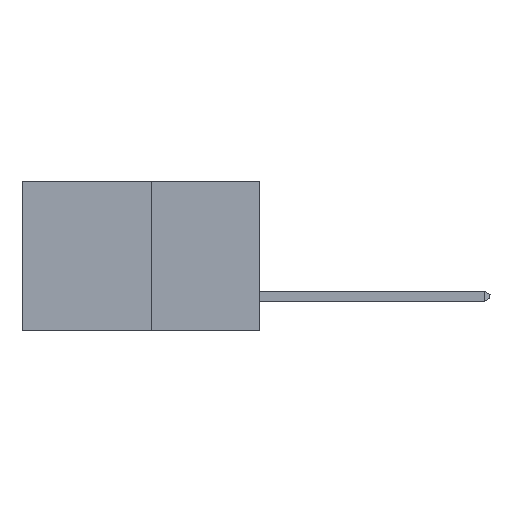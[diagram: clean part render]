
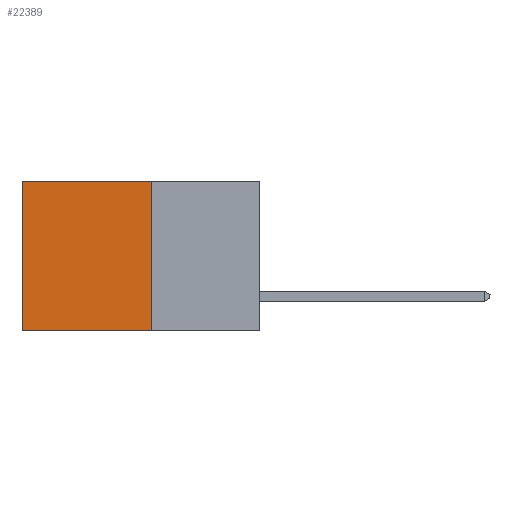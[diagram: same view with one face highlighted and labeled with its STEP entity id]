
A CAD part, left-side view. The second image highlights one B-rep face of the part: STEP entity #22389.
In plain terms, the highlighted planar face has unit normal (-1, 0, 0).
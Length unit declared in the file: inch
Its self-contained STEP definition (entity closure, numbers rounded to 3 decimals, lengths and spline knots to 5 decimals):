
#35 = EDGE_CURVE ( 'NONE', #2760, #16097, #5127, .T. ) ;
#55 = VECTOR ( 'NONE', #8610, 39.37008 ) ;
#414 = ORIENTED_EDGE ( 'NONE', *, *, #6841, .T. ) ;
#1890 = FACE_OUTER_BOUND ( 'NONE', #8741, .T. ) ;
#1989 = DIRECTION ( 'NONE',  ( 0., 0., -1. ) ) ;
#2028 = CARTESIAN_POINT ( 'NONE',  ( 0.277, 0.27, -0.37 ) ) ;
#2065 = CARTESIAN_POINT ( 'NONE',  ( 0.277, 0.27, -0.37 ) ) ;
#2424 = ORIENTED_EDGE ( 'NONE', *, *, #10215, .F. ) ;
#2492 = VERTEX_POINT ( 'NONE', #2028 ) ;
#2760 = VERTEX_POINT ( 'NONE', #15200 ) ;
#5027 = CARTESIAN_POINT ( 'NONE',  ( 0.277, 0.27, 0. ) ) ;
#5127 = LINE ( 'NONE', #5027, #17813 ) ;
#5562 = AXIS2_PLACEMENT_3D ( 'NONE', #21524, #6050, #18117 ) ;
#6050 = DIRECTION ( 'NONE',  ( 1., 0., 0. ) ) ;
#6537 = ORIENTED_EDGE ( 'NONE', *, *, #35, .T. ) ;
#6841 = EDGE_CURVE ( 'NONE', #16097, #18708, #19051, .T. ) ;
#8126 = DIRECTION ( 'NONE',  ( 0., 0., -1. ) ) ;
#8457 = EDGE_CURVE ( 'NONE', #2760, #2492, #14394, .T. ) ;
#8610 = DIRECTION ( 'NONE',  ( 0., 1., 0. ) ) ;
#8741 = EDGE_LOOP ( 'NONE', ( #414, #2424, #16167, #6537 ) ) ;
#9827 = VECTOR ( 'NONE', #1989, 39.37008 ) ;
#10215 = EDGE_CURVE ( 'NONE', #2492, #18708, #13925, .T. ) ;
#11224 = PLANE ( 'NONE',  #5562 ) ;
#11550 = CARTESIAN_POINT ( 'NONE',  ( 0.277, 0.59, -0.37 ) ) ;
#13876 = CARTESIAN_POINT ( 'NONE',  ( 0.277, 0.59, -0.37 ) ) ;
#13925 = LINE ( 'NONE', #17156, #55 ) ;
#14394 = LINE ( 'NONE', #2065, #9827 ) ;
#14451 = VECTOR ( 'NONE', #8126, 39.37008 ) ;
#15200 = CARTESIAN_POINT ( 'NONE',  ( 0.277, 0.27, 0. ) ) ;
#15879 = CARTESIAN_POINT ( 'NONE',  ( 0.277, 0.59, 0. ) ) ;
#16097 = VERTEX_POINT ( 'NONE', #15879 ) ;
#16167 = ORIENTED_EDGE ( 'NONE', *, *, #8457, .F. ) ;
#17156 = CARTESIAN_POINT ( 'NONE',  ( 0.277, 0.27, -0.37 ) ) ;
#17813 = VECTOR ( 'NONE', #18679, 39.37008 ) ;
#18117 = DIRECTION ( 'NONE',  ( 0., 0., -1. ) ) ;
#18679 = DIRECTION ( 'NONE',  ( 0., 1., 0. ) ) ;
#18708 = VERTEX_POINT ( 'NONE', #13876 ) ;
#19051 = LINE ( 'NONE', #11550, #14451 ) ;
#21524 = CARTESIAN_POINT ( 'NONE',  ( 0.277, 0.27, -0.37 ) ) ;
#22389 = ADVANCED_FACE ( 'NONE', ( #1890 ), #11224, .F. ) ;
